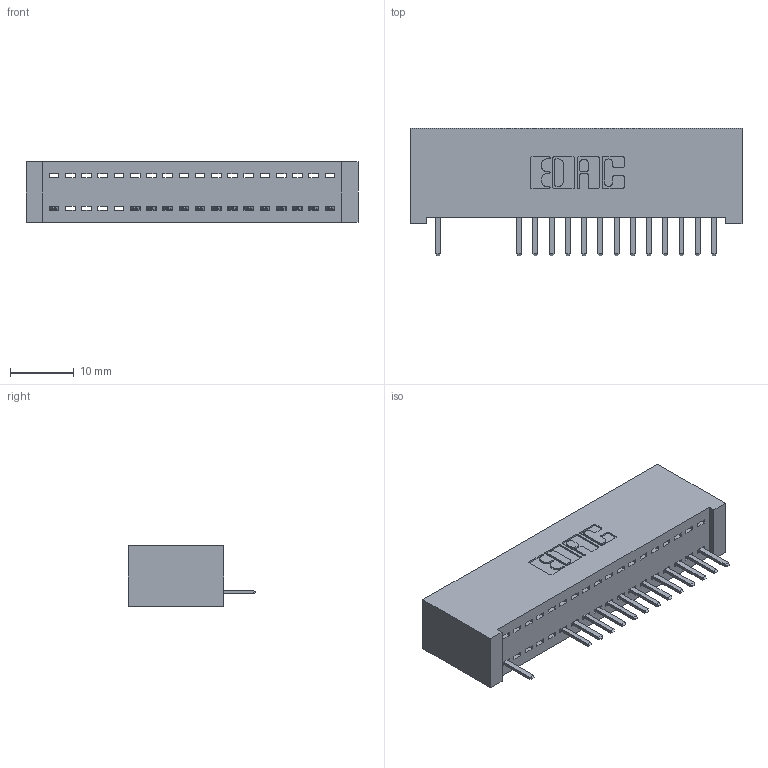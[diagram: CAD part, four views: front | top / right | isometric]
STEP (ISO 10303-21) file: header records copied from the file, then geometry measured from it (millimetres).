
FILE_DESCRIPTION (( 'STEP AP203' ), '1' );
FILE_NAME ('392-018-520-101.STEP', '2018-08-15T03:29:37', ( '' ), ( '' ), 'SwSTEP 2.0', 'SolidWorks 2016', '' );
FILE_SCHEMA (( 'CONFIG_CONTROL_DESIGN' ));
Length unit declared in the file: inch
Products named in the file (3): 342 Part_Lugless; 345-292-001_345-293-120; 392-018-520-101
Assembly tree (15 placements, depth 2):
  392-018-520-101
    342 Part_Lugless
    345-292-001_345-293-120  x14
Bounding box: 51.97 x 20.02 x 9.4 mm (x, y, z)
Volume: 4791.1 mm3; surface area: 6544.9 mm2
Topology: 15 solids, 15 shells, 1018 faces, 3019 edges, 1974 vertices
Faces by surface type: plane 726, cylinder 292
Entity records: 13685 total; most frequent: CARTESIAN_POINT 2400, ORIENTED_EDGE 2346, DIRECTION 2049, EDGE_CURVE 1173, LINE 1049, VECTOR 1049, VERTEX_POINT 778, AXIS2_PLACEMENT_3D 500
